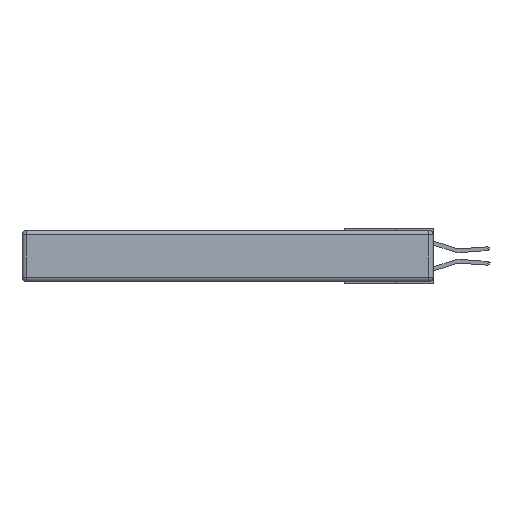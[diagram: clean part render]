
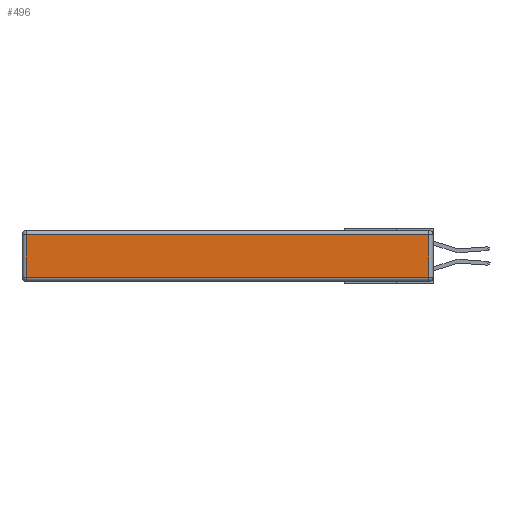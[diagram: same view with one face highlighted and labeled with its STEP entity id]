
A CAD part, left-side view. The second image highlights one B-rep face of the part: STEP entity #496.
In plain terms, the highlighted planar face has unit normal (-1, 0, 0).
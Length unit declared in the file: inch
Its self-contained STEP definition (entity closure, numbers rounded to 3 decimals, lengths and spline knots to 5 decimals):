
#171 = CARTESIAN_POINT ( 'NONE',  ( 0., 2.72, -0.343 ) ) ;
#260 = ORIENTED_EDGE ( 'NONE', *, *, #6924, .T. ) ;
#371 = VECTOR ( 'NONE', #13363, 39.37008 ) ;
#496 = ADVANCED_FACE ( 'NONE', ( #14695 ), #5667, .T. ) ;
#756 = EDGE_CURVE ( 'NONE', #1466, #4169, #14881, .T. ) ;
#1466 = VERTEX_POINT ( 'NONE', #15960 ) ;
#3293 = DIRECTION ( 'NONE',  ( 0., 0., 1. ) ) ;
#3982 = CARTESIAN_POINT ( 'NONE',  ( 0., 2.72, -0.03 ) ) ;
#4169 = VERTEX_POINT ( 'NONE', #7689 ) ;
#5209 = VECTOR ( 'NONE', #3293, 39.37008 ) ;
#5241 = VERTEX_POINT ( 'NONE', #14546 ) ;
#5258 = EDGE_CURVE ( 'NONE', #5241, #1466, #14496, .T. ) ;
#5567 = VECTOR ( 'NONE', #14539, 39.37008 ) ;
#5667 = PLANE ( 'NONE',  #13128 ) ;
#6924 = EDGE_CURVE ( 'NONE', #13313, #5241, #9026, .T. ) ;
#7045 = DIRECTION ( 'NONE',  ( 0., 0., 1. ) ) ;
#7689 = CARTESIAN_POINT ( 'NONE',  ( 0., 0.03, -0.03 ) ) ;
#8115 = CARTESIAN_POINT ( 'NONE',  ( 0., 0.03, -0.343 ) ) ;
#8186 = CARTESIAN_POINT ( 'NONE',  ( 0., 0., -0.343 ) ) ;
#8751 = EDGE_CURVE ( 'NONE', #4169, #13313, #12157, .T. ) ;
#9026 = LINE ( 'NONE', #171, #5567 ) ;
#9735 = ORIENTED_EDGE ( 'NONE', *, *, #8751, .T. ) ;
#10167 = VECTOR ( 'NONE', #16266, 39.37008 ) ;
#10987 = CARTESIAN_POINT ( 'NONE',  ( 0., 2.75, -0.03 ) ) ;
#11709 = EDGE_LOOP ( 'NONE', ( #12810, #12814, #9735, #260 ) ) ;
#12157 = LINE ( 'NONE', #10987, #10167 ) ;
#12810 = ORIENTED_EDGE ( 'NONE', *, *, #5258, .T. ) ;
#12814 = ORIENTED_EDGE ( 'NONE', *, *, #756, .T. ) ;
#13128 = AXIS2_PLACEMENT_3D ( 'NONE', #8186, #16102, #7045 ) ;
#13313 = VERTEX_POINT ( 'NONE', #3982 ) ;
#13316 = CARTESIAN_POINT ( 'NONE',  ( 0., 0., -0.313 ) ) ;
#13363 = DIRECTION ( 'NONE',  ( 0., -1., 0. ) ) ;
#14496 = LINE ( 'NONE', #13316, #371 ) ;
#14539 = DIRECTION ( 'NONE',  ( 0., 0., -1. ) ) ;
#14546 = CARTESIAN_POINT ( 'NONE',  ( 0., 2.72, -0.313 ) ) ;
#14695 = FACE_OUTER_BOUND ( 'NONE', #11709, .T. ) ;
#14881 = LINE ( 'NONE', #8115, #5209 ) ;
#15960 = CARTESIAN_POINT ( 'NONE',  ( 0., 0.03, -0.313 ) ) ;
#16102 = DIRECTION ( 'NONE',  ( -1., 0., 0. ) ) ;
#16266 = DIRECTION ( 'NONE',  ( 0., 1., 0. ) ) ;
